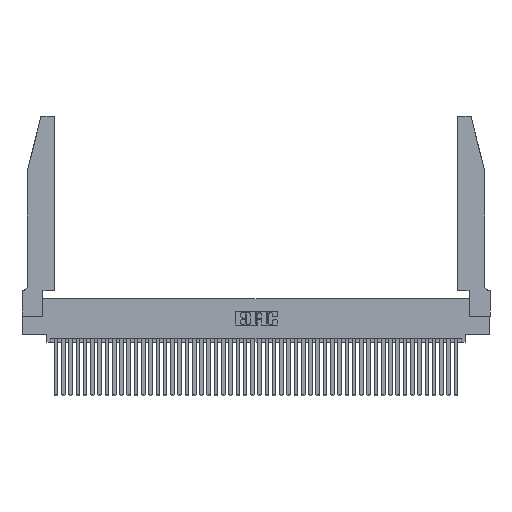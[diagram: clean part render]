
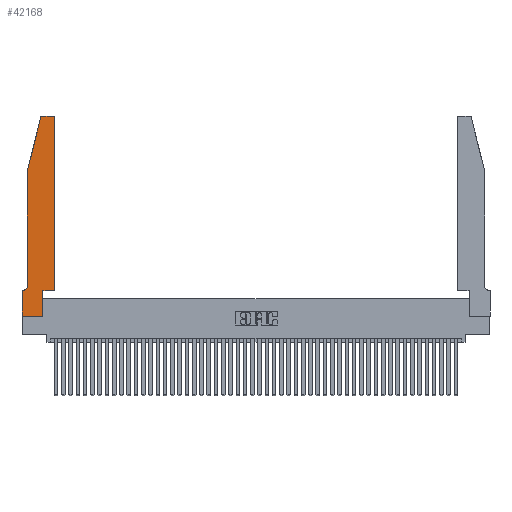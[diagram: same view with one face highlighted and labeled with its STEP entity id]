
A CAD part, top view. The second image highlights one B-rep face of the part: STEP entity #42168.
In plain terms, the highlighted planar face has unit normal (0, 0, 1).
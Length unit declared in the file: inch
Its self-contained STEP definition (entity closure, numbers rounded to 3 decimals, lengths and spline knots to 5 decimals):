
#269 = VECTOR ( 'NONE', #20960, 39.37008 ) ;
#684 = VECTOR ( 'NONE', #24817, 39.37008 ) ;
#971 = VERTEX_POINT ( 'NONE', #13838 ) ;
#1436 = LINE ( 'NONE', #15420, #22952 ) ;
#1586 = DIRECTION ( 'NONE',  ( -1., 0., 0. ) ) ;
#2488 = VERTEX_POINT ( 'NONE', #17285 ) ;
#2489 = VERTEX_POINT ( 'NONE', #9566 ) ;
#2561 = CARTESIAN_POINT ( 'NONE',  ( 0.4505, 0.35, 0.37 ) ) ;
#2709 = DIRECTION ( 'NONE',  ( 1., 0., 0. ) ) ;
#2748 = VERTEX_POINT ( 'NONE', #20013 ) ;
#3061 = ORIENTED_EDGE ( 'NONE', *, *, #6603, .T. ) ;
#5035 = EDGE_CURVE ( 'NONE', #6665, #2748, #5438, .T. ) ;
#5206 = CARTESIAN_POINT ( 'NONE',  ( 0.284, 2.75, 0.37 ) ) ;
#5438 = CIRCLE ( 'NONE', #13638, 0.07 ) ;
#5441 = DIRECTION ( 'NONE',  ( 1., 0., 0. ) ) ;
#5591 = DIRECTION ( 'NONE',  ( 0., 0., 1. ) ) ;
#6603 = EDGE_CURVE ( 'NONE', #33231, #15427, #16590, .T. ) ;
#6665 = VERTEX_POINT ( 'NONE', #38791 ) ;
#6666 = CIRCLE ( 'NONE', #15293, 0.03 ) ;
#6738 = CARTESIAN_POINT ( 'NONE',  ( 0., 0.35, 0.37 ) ) ;
#7856 = LINE ( 'NONE', #32195, #14143 ) ;
#8076 = LINE ( 'NONE', #42115, #16085 ) ;
#8284 = DIRECTION ( 'NONE',  ( 0., -1., 0. ) ) ;
#9566 = CARTESIAN_POINT ( 'NONE',  ( 0.0755, 2., 0.37 ) ) ;
#9900 = DIRECTION ( 'NONE',  ( 0., 0., 1. ) ) ;
#9928 = ORIENTED_EDGE ( 'NONE', *, *, #5035, .T. ) ;
#9961 = DIRECTION ( 'NONE',  ( 0., 0., 1. ) ) ;
#10065 = VERTEX_POINT ( 'NONE', #39952 ) ;
#10382 = ORIENTED_EDGE ( 'NONE', *, *, #22942, .T. ) ;
#10644 = ORIENTED_EDGE ( 'NONE', *, *, #22237, .T. ) ;
#11084 = ORIENTED_EDGE ( 'NONE', *, *, #24423, .T. ) ;
#12045 = ORIENTED_EDGE ( 'NONE', *, *, #34525, .T. ) ;
#12175 = LINE ( 'NONE', #41255, #18911 ) ;
#12293 = EDGE_CURVE ( 'NONE', #2488, #971, #27593, .T. ) ;
#13638 = AXIS2_PLACEMENT_3D ( 'NONE', #37814, #30388, #1586 ) ;
#13838 = CARTESIAN_POINT ( 'NONE',  ( 0.4505, 2.72, 0.37 ) ) ;
#14143 = VECTOR ( 'NONE', #24518, 39.37008 ) ;
#14419 = EDGE_LOOP ( 'NONE', ( #3061, #26170, #11084, #10644, #9928, #12045, #20714, #40190, #10382, #20514, #42686, #43737 ) ) ;
#15293 = AXIS2_PLACEMENT_3D ( 'NONE', #30595, #5591, #5441 ) ;
#15420 = CARTESIAN_POINT ( 'NONE',  ( 0.0755, 2., 0.37 ) ) ;
#15427 = VERTEX_POINT ( 'NONE', #5206 ) ;
#16085 = VECTOR ( 'NONE', #19995, 39.37008 ) ;
#16590 = LINE ( 'NONE', #39582, #684 ) ;
#17285 = CARTESIAN_POINT ( 'NONE',  ( 0.4505, 0.35, 0.37 ) ) ;
#18109 = VERTEX_POINT ( 'NONE', #31231 ) ;
#18911 = VECTOR ( 'NONE', #45229, 39.37008 ) ;
#19995 = DIRECTION ( 'NONE',  ( -1., 0., 0. ) ) ;
#20013 = CARTESIAN_POINT ( 'NONE',  ( 0.0055, 0.35, 0.37 ) ) ;
#20401 = CARTESIAN_POINT ( 'NONE',  ( 0., 0.35, 0.37 ) ) ;
#20514 = ORIENTED_EDGE ( 'NONE', *, *, #30073, .T. ) ;
#20519 = VERTEX_POINT ( 'NONE', #22631 ) ;
#20714 = ORIENTED_EDGE ( 'NONE', *, *, #36650, .T. ) ;
#20960 = DIRECTION ( 'NONE',  ( 0., 1., 0. ) ) ;
#21863 = AXIS2_PLACEMENT_3D ( 'NONE', #20401, #9961, #2709 ) ;
#22237 = EDGE_CURVE ( 'NONE', #2489, #6665, #1436, .T. ) ;
#22631 = CARTESIAN_POINT ( 'NONE',  ( 0.25487, 2.72718, 0.37 ) ) ;
#22888 = EDGE_CURVE ( 'NONE', #971, #33231, #26893, .T. ) ;
#22942 = EDGE_CURVE ( 'NONE', #39853, #18109, #28559, .T. ) ;
#22952 = VECTOR ( 'NONE', #8284, 39.37008 ) ;
#24085 = CARTESIAN_POINT ( 'NONE',  ( 0.4205, 2.75, 0.37 ) ) ;
#24423 = EDGE_CURVE ( 'NONE', #20519, #2489, #31262, .T. ) ;
#24518 = DIRECTION ( 'NONE',  ( 0., -1., 0. ) ) ;
#24763 = CARTESIAN_POINT ( 'NONE',  ( 0.4205, 2.72, 0.37 ) ) ;
#24817 = DIRECTION ( 'NONE',  ( -1., 0., 0. ) ) ;
#26170 = ORIENTED_EDGE ( 'NONE', *, *, #27978, .T. ) ;
#26893 = CIRCLE ( 'NONE', #43213, 0.03 ) ;
#27593 = LINE ( 'NONE', #2561, #42244 ) ;
#27978 = EDGE_CURVE ( 'NONE', #15427, #20519, #6666, .T. ) ;
#28559 = LINE ( 'NONE', #45954, #269 ) ;
#30073 = EDGE_CURVE ( 'NONE', #18109, #2488, #12175, .T. ) ;
#30388 = DIRECTION ( 'NONE',  ( 0., 0., -1. ) ) ;
#30595 = CARTESIAN_POINT ( 'NONE',  ( 0.284, 2.72, 0.37 ) ) ;
#30631 = VECTOR ( 'NONE', #31222, 39.37008 ) ;
#31222 = DIRECTION ( 'NONE',  ( 1., 0., 0. ) ) ;
#31231 = CARTESIAN_POINT ( 'NONE',  ( 0.2865, 0.35, 0.37 ) ) ;
#31262 = LINE ( 'NONE', #33793, #31806 ) ;
#31806 = VECTOR ( 'NONE', #44716, 39.37008 ) ;
#31861 = FACE_OUTER_BOUND ( 'NONE', #14419, .T. ) ;
#32195 = CARTESIAN_POINT ( 'NONE',  ( 0., 0., 0.37 ) ) ;
#33231 = VERTEX_POINT ( 'NONE', #24085 ) ;
#33793 = CARTESIAN_POINT ( 'NONE',  ( 0.0755, 2., 0.37 ) ) ;
#34018 = VERTEX_POINT ( 'NONE', #6738 ) ;
#34525 = EDGE_CURVE ( 'NONE', #2748, #34018, #8076, .T. ) ;
#36650 = EDGE_CURVE ( 'NONE', #34018, #10065, #7856, .T. ) ;
#36789 = LINE ( 'NONE', #38151, #30631 ) ;
#36863 = CARTESIAN_POINT ( 'NONE',  ( 0.2865, 0., 0.37 ) ) ;
#37814 = CARTESIAN_POINT ( 'NONE',  ( 0.0055, 0.42, 0.37 ) ) ;
#38151 = CARTESIAN_POINT ( 'NONE',  ( 0., 0., 0.37 ) ) ;
#38676 = DIRECTION ( 'NONE',  ( 1., 0., 0. ) ) ;
#38735 = PLANE ( 'NONE',  #21863 ) ;
#38791 = CARTESIAN_POINT ( 'NONE',  ( 0.0755, 0.42, 0.37 ) ) ;
#39582 = CARTESIAN_POINT ( 'NONE',  ( 0.2605, 2.75, 0.37 ) ) ;
#39853 = VERTEX_POINT ( 'NONE', #36863 ) ;
#39952 = CARTESIAN_POINT ( 'NONE',  ( 0., 0., 0.37 ) ) ;
#40190 = ORIENTED_EDGE ( 'NONE', *, *, #43557, .T. ) ;
#41255 = CARTESIAN_POINT ( 'NONE',  ( 0.4505, 0.35, 0.37 ) ) ;
#42115 = CARTESIAN_POINT ( 'NONE',  ( 0.0755, 0.35, 0.37 ) ) ;
#42168 = ADVANCED_FACE ( 'NONE', ( #31861 ), #38735, .T. ) ;
#42244 = VECTOR ( 'NONE', #43690, 39.37008 ) ;
#42686 = ORIENTED_EDGE ( 'NONE', *, *, #12293, .T. ) ;
#43213 = AXIS2_PLACEMENT_3D ( 'NONE', #24763, #9900, #38676 ) ;
#43557 = EDGE_CURVE ( 'NONE', #10065, #39853, #36789, .T. ) ;
#43690 = DIRECTION ( 'NONE',  ( 0., 1., 0. ) ) ;
#43737 = ORIENTED_EDGE ( 'NONE', *, *, #22888, .T. ) ;
#44716 = DIRECTION ( 'NONE',  ( -0.239, -0.971, 0. ) ) ;
#45229 = DIRECTION ( 'NONE',  ( 1., 0., 0. ) ) ;
#45954 = CARTESIAN_POINT ( 'NONE',  ( 0.2865, 0.35, 0.37 ) ) ;
